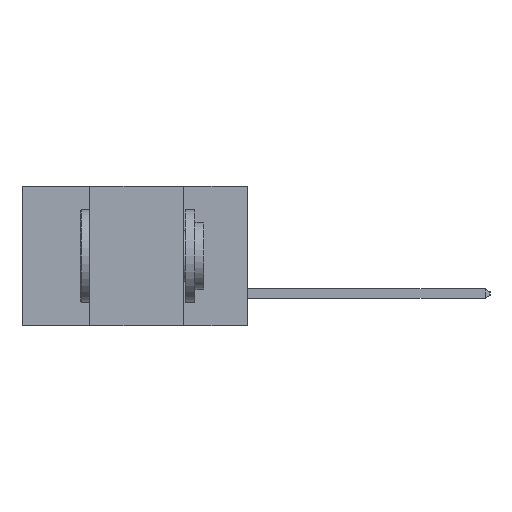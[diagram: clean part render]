
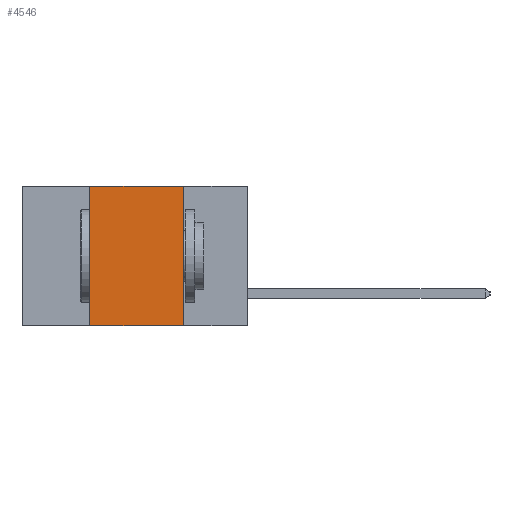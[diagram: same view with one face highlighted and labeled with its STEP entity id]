
A CAD part, left-side view. The second image highlights one B-rep face of the part: STEP entity #4546.
In plain terms, the highlighted planar face has unit normal (-1, 0, 0).
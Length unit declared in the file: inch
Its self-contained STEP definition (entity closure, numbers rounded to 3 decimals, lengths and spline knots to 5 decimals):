
#302 = AXIS2_PLACEMENT_3D ( 'NONE', #909, #20095, #19925 ) ;
#909 = CARTESIAN_POINT ( 'NONE',  ( 0., 0.6, 0. ) ) ;
#2516 = DIRECTION ( 'NONE',  ( 0., 0., 1. ) ) ;
#2604 = CARTESIAN_POINT ( 'NONE',  ( 0., 0.42, 0. ) ) ;
#3035 = EDGE_CURVE ( 'NONE', #13752, #19174, #18497, .T. ) ;
#3339 = CARTESIAN_POINT ( 'NONE',  ( 0., 0.42, -0.37 ) ) ;
#3451 = EDGE_CURVE ( 'NONE', #19174, #8399, #19016, .T. ) ;
#4241 = VECTOR ( 'NONE', #17787, 39.37008 ) ;
#4546 = ADVANCED_FACE ( 'NONE', ( #11416 ), #20172, .F. ) ;
#5219 = VECTOR ( 'NONE', #20645, 39.37008 ) ;
#5334 = EDGE_CURVE ( 'NONE', #13752, #15509, #13568, .T. ) ;
#7745 = ORIENTED_EDGE ( 'NONE', *, *, #3451, .F. ) ;
#8399 = VERTEX_POINT ( 'NONE', #15922 ) ;
#11416 = FACE_OUTER_BOUND ( 'NONE', #21398, .T. ) ;
#11517 = DIRECTION ( 'NONE',  ( 0., 0., -1. ) ) ;
#11822 = ORIENTED_EDGE ( 'NONE', *, *, #5334, .T. ) ;
#12294 = CARTESIAN_POINT ( 'NONE',  ( 0., 0.17, -0.37 ) ) ;
#12353 = ORIENTED_EDGE ( 'NONE', *, *, #15555, .F. ) ;
#13139 = VECTOR ( 'NONE', #11517, 39.37008 ) ;
#13371 = CARTESIAN_POINT ( 'NONE',  ( 0., 0.17, -0.37 ) ) ;
#13568 = LINE ( 'NONE', #17882, #4241 ) ;
#13752 = VERTEX_POINT ( 'NONE', #14844 ) ;
#14017 = VECTOR ( 'NONE', #2516, 39.37008 ) ;
#14844 = CARTESIAN_POINT ( 'NONE',  ( 0., 0.42, -0.37 ) ) ;
#15509 = VERTEX_POINT ( 'NONE', #13371 ) ;
#15555 = EDGE_CURVE ( 'NONE', #8399, #15509, #17648, .T. ) ;
#15922 = CARTESIAN_POINT ( 'NONE',  ( 0., 0.17, 0. ) ) ;
#16380 = ORIENTED_EDGE ( 'NONE', *, *, #3035, .F. ) ;
#17648 = LINE ( 'NONE', #12294, #13139 ) ;
#17787 = DIRECTION ( 'NONE',  ( 0., -1., 0. ) ) ;
#17882 = CARTESIAN_POINT ( 'NONE',  ( 0., 0.6, -0.37 ) ) ;
#18497 = LINE ( 'NONE', #3339, #14017 ) ;
#19016 = LINE ( 'NONE', #20879, #5219 ) ;
#19174 = VERTEX_POINT ( 'NONE', #2604 ) ;
#19925 = DIRECTION ( 'NONE',  ( 0., 0., -1. ) ) ;
#20095 = DIRECTION ( 'NONE',  ( 1., 0., 0. ) ) ;
#20172 = PLANE ( 'NONE',  #302 ) ;
#20645 = DIRECTION ( 'NONE',  ( 0., -1., 0. ) ) ;
#20879 = CARTESIAN_POINT ( 'NONE',  ( 0., 0.6, 0. ) ) ;
#21398 = EDGE_LOOP ( 'NONE', ( #12353, #7745, #16380, #11822 ) ) ;
